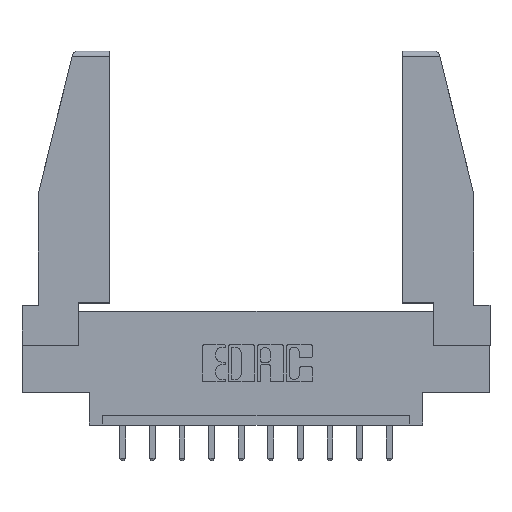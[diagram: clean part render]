
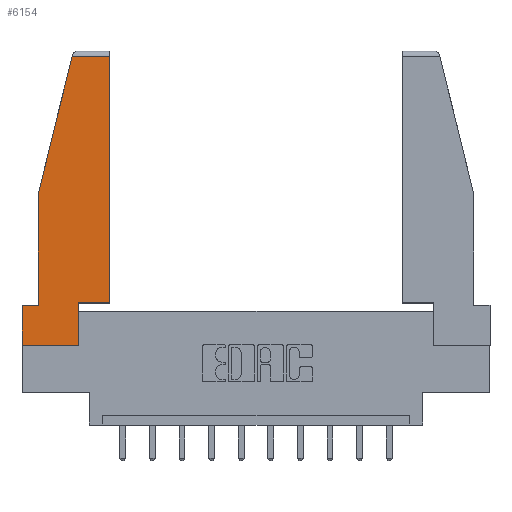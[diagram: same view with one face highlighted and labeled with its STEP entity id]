
A CAD part, top view. The second image highlights one B-rep face of the part: STEP entity #6154.
In plain terms, the highlighted planar face has unit normal (0, 0, 1).
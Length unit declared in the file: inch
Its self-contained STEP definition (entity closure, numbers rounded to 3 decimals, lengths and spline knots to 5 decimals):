
#199 = DIRECTION ( 'NONE',  ( -0.239, -0.971, 0. ) ) ;
#264 = CARTESIAN_POINT ( 'NONE',  ( 0.086, 0.21, 0. ) ) ;
#278 = CARTESIAN_POINT ( 'NONE',  ( 0.297, 0.223, 0. ) ) ;
#364 = EDGE_LOOP ( 'NONE', ( #13906, #6380, #13006, #5301, #2715, #5183, #8613, #2528, #7920 ) ) ;
#508 = DIRECTION ( 'NONE',  ( 0., 1., 0. ) ) ;
#644 = VECTOR ( 'NONE', #13177, 39.37008 ) ;
#670 = LINE ( 'NONE', #2617, #3242 ) ;
#734 = DIRECTION ( 'NONE',  ( 1., 0., 0. ) ) ;
#1037 = CARTESIAN_POINT ( 'NONE',  ( 0.461, 1.52, 0. ) ) ;
#1301 = CARTESIAN_POINT ( 'NONE',  ( 0., 1.52, 0. ) ) ;
#2372 = CARTESIAN_POINT ( 'NONE',  ( 0.086, 0.8, 0. ) ) ;
#2450 = CARTESIAN_POINT ( 'NONE',  ( 0.271, 1.55, 0. ) ) ;
#2528 = ORIENTED_EDGE ( 'NONE', *, *, #5717, .T. ) ;
#2550 = VERTEX_POINT ( 'NONE', #9252 ) ;
#2617 = CARTESIAN_POINT ( 'NONE',  ( 0., 0.21, 0. ) ) ;
#2683 = VERTEX_POINT ( 'NONE', #11611 ) ;
#2710 = CARTESIAN_POINT ( 'NONE',  ( 0., 0., 0. ) ) ;
#2715 = ORIENTED_EDGE ( 'NONE', *, *, #7349, .T. ) ;
#2868 = EDGE_CURVE ( 'NONE', #4887, #7658, #9758, .T. ) ;
#3242 = VECTOR ( 'NONE', #11211, 39.37008 ) ;
#3516 = VECTOR ( 'NONE', #9043, 39.37008 ) ;
#3804 = VECTOR ( 'NONE', #508, 39.37008 ) ;
#3992 = CARTESIAN_POINT ( 'NONE',  ( 0., 0., 0. ) ) ;
#4234 = LINE ( 'NONE', #2710, #644 ) ;
#4324 = DIRECTION ( 'NONE',  ( 0., 1., 0. ) ) ;
#4772 = CARTESIAN_POINT ( 'NONE',  ( 0.086, 0.8, 0. ) ) ;
#4887 = VERTEX_POINT ( 'NONE', #6267 ) ;
#4997 = LINE ( 'NONE', #1301, #10873 ) ;
#5159 = VERTEX_POINT ( 'NONE', #1037 ) ;
#5183 = ORIENTED_EDGE ( 'NONE', *, *, #2868, .T. ) ;
#5301 = ORIENTED_EDGE ( 'NONE', *, *, #7711, .T. ) ;
#5382 = VERTEX_POINT ( 'NONE', #4772 ) ;
#5717 = EDGE_CURVE ( 'NONE', #2683, #5889, #12572, .T. ) ;
#5889 = VERTEX_POINT ( 'NONE', #10137 ) ;
#6154 = ADVANCED_FACE ( 'NONE', ( #10704 ), #9368, .T. ) ;
#6267 = CARTESIAN_POINT ( 'NONE',  ( 0., 0.21, 0. ) ) ;
#6380 = ORIENTED_EDGE ( 'NONE', *, *, #12060, .T. ) ;
#6478 = LINE ( 'NONE', #278, #8207 ) ;
#6892 = CARTESIAN_POINT ( 'NONE',  ( 0.461, 0.223, 0. ) ) ;
#7349 = EDGE_CURVE ( 'NONE', #11541, #4887, #670, .T. ) ;
#7658 = VERTEX_POINT ( 'NONE', #12324 ) ;
#7707 = EDGE_CURVE ( 'NONE', #5889, #11140, #6478, .T. ) ;
#7711 = EDGE_CURVE ( 'NONE', #5382, #11541, #12350, .T. ) ;
#7784 = EDGE_CURVE ( 'NONE', #7658, #2683, #4234, .T. ) ;
#7920 = ORIENTED_EDGE ( 'NONE', *, *, #7707, .T. ) ;
#8207 = VECTOR ( 'NONE', #13389, 39.37008 ) ;
#8613 = ORIENTED_EDGE ( 'NONE', *, *, #7784, .T. ) ;
#8621 = LINE ( 'NONE', #2450, #11214 ) ;
#8996 = DIRECTION ( 'NONE',  ( 0., -1., 0. ) ) ;
#9043 = DIRECTION ( 'NONE',  ( 0., -1., 0. ) ) ;
#9252 = CARTESIAN_POINT ( 'NONE',  ( 0.2636, 1.52, 0. ) ) ;
#9368 = PLANE ( 'NONE',  #11239 ) ;
#9758 = LINE ( 'NONE', #10114, #3516 ) ;
#9789 = VECTOR ( 'NONE', #8996, 39.37008 ) ;
#10114 = CARTESIAN_POINT ( 'NONE',  ( 0., 0.21, 0. ) ) ;
#10137 = CARTESIAN_POINT ( 'NONE',  ( 0.297, 0.223, 0. ) ) ;
#10542 = LINE ( 'NONE', #6892, #3804 ) ;
#10704 = FACE_OUTER_BOUND ( 'NONE', #364, .T. ) ;
#10873 = VECTOR ( 'NONE', #11342, 39.37008 ) ;
#10958 = CARTESIAN_POINT ( 'NONE',  ( 0.297, 0., 0. ) ) ;
#11140 = VERTEX_POINT ( 'NONE', #14112 ) ;
#11211 = DIRECTION ( 'NONE',  ( -1., 0., 0. ) ) ;
#11214 = VECTOR ( 'NONE', #199, 39.37008 ) ;
#11215 = VECTOR ( 'NONE', #4324, 39.37008 ) ;
#11239 = AXIS2_PLACEMENT_3D ( 'NONE', #3992, #11523, #734 ) ;
#11342 = DIRECTION ( 'NONE',  ( -1., 0., 0. ) ) ;
#11523 = DIRECTION ( 'NONE',  ( 0., 0., 1. ) ) ;
#11541 = VERTEX_POINT ( 'NONE', #264 ) ;
#11580 = EDGE_CURVE ( 'NONE', #11140, #5159, #10542, .T. ) ;
#11611 = CARTESIAN_POINT ( 'NONE',  ( 0.297, 0., 0. ) ) ;
#12057 = EDGE_CURVE ( 'NONE', #2550, #5382, #8621, .T. ) ;
#12060 = EDGE_CURVE ( 'NONE', #5159, #2550, #4997, .T. ) ;
#12324 = CARTESIAN_POINT ( 'NONE',  ( 0., 0., 0. ) ) ;
#12350 = LINE ( 'NONE', #2372, #9789 ) ;
#12572 = LINE ( 'NONE', #10958, #11215 ) ;
#13006 = ORIENTED_EDGE ( 'NONE', *, *, #12057, .T. ) ;
#13177 = DIRECTION ( 'NONE',  ( 1., 0., 0. ) ) ;
#13389 = DIRECTION ( 'NONE',  ( 1., 0., 0. ) ) ;
#13906 = ORIENTED_EDGE ( 'NONE', *, *, #11580, .T. ) ;
#14112 = CARTESIAN_POINT ( 'NONE',  ( 0.461, 0.223, 0. ) ) ;
